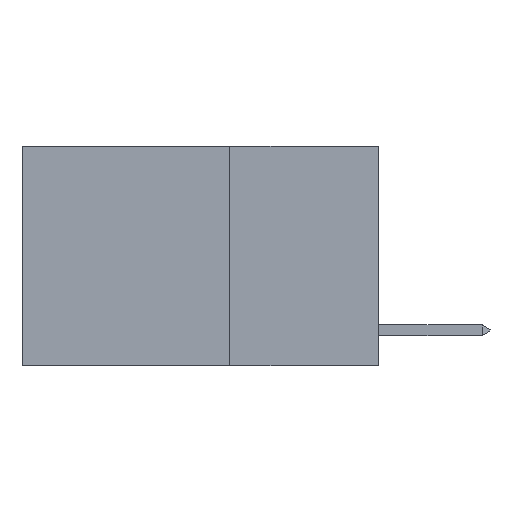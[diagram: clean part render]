
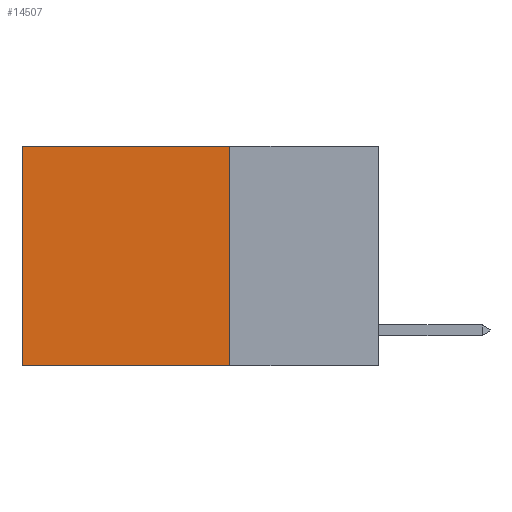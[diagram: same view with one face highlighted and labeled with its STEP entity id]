
A CAD part, left-side view. The second image highlights one B-rep face of the part: STEP entity #14507.
In plain terms, the highlighted planar face has unit normal (-1, 0, 0).
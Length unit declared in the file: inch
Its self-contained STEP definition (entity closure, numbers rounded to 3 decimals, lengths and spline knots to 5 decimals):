
#401 = DIRECTION ( 'NONE',  ( 0., 1., 0. ) ) ;
#1556 = ORIENTED_EDGE ( 'NONE', *, *, #18446, .T. ) ;
#2147 = CARTESIAN_POINT ( 'NONE',  ( 0.2625, 0.25, 0. ) ) ;
#2982 = VERTEX_POINT ( 'NONE', #14710 ) ;
#4727 = CARTESIAN_POINT ( 'NONE',  ( 0.2625, 0.25, -0.37 ) ) ;
#6183 = ORIENTED_EDGE ( 'NONE', *, *, #27543, .T. ) ;
#8913 = CARTESIAN_POINT ( 'NONE',  ( 0.2625, 0.25, 0. ) ) ;
#9107 = VECTOR ( 'NONE', #10740, 39.37008 ) ;
#9133 = LINE ( 'NONE', #17726, #14796 ) ;
#10447 = CARTESIAN_POINT ( 'NONE',  ( 0.2625, 0.6, 0. ) ) ;
#10517 = EDGE_CURVE ( 'NONE', #2982, #15190, #16819, .T. ) ;
#10740 = DIRECTION ( 'NONE',  ( 0., 1., 0. ) ) ;
#11075 = DIRECTION ( 'NONE',  ( 0., 0., -1. ) ) ;
#11199 = VECTOR ( 'NONE', #13147, 39.37008 ) ;
#11782 = ORIENTED_EDGE ( 'NONE', *, *, #15680, .F. ) ;
#12975 = LINE ( 'NONE', #10447, #17911 ) ;
#13147 = DIRECTION ( 'NONE',  ( 0., 0., -1. ) ) ;
#14507 = ADVANCED_FACE ( 'NONE', ( #14511 ), #19463, .F. ) ;
#14511 = FACE_OUTER_BOUND ( 'NONE', #19646, .T. ) ;
#14710 = CARTESIAN_POINT ( 'NONE',  ( 0.2625, 0.25, 0. ) ) ;
#14771 = LINE ( 'NONE', #19138, #9107 ) ;
#14796 = VECTOR ( 'NONE', #401, 39.37008 ) ;
#15190 = VERTEX_POINT ( 'NONE', #4727 ) ;
#15680 = EDGE_CURVE ( 'NONE', #15190, #26964, #14771, .T. ) ;
#16819 = LINE ( 'NONE', #2147, #11199 ) ;
#17726 = CARTESIAN_POINT ( 'NONE',  ( 0.2625, 0.25, 0. ) ) ;
#17911 = VECTOR ( 'NONE', #18948, 39.37008 ) ;
#18446 = EDGE_CURVE ( 'NONE', #2982, #23501, #9133, .T. ) ;
#18948 = DIRECTION ( 'NONE',  ( 0., 0., -1. ) ) ;
#19138 = CARTESIAN_POINT ( 'NONE',  ( 0.2625, 0.25, -0.37 ) ) ;
#19463 = PLANE ( 'NONE',  #19617 ) ;
#19617 = AXIS2_PLACEMENT_3D ( 'NONE', #8913, #23607, #11075 ) ;
#19646 = EDGE_LOOP ( 'NONE', ( #6183, #11782, #19847, #1556 ) ) ;
#19847 = ORIENTED_EDGE ( 'NONE', *, *, #10517, .F. ) ;
#23501 = VERTEX_POINT ( 'NONE', #27361 ) ;
#23607 = DIRECTION ( 'NONE',  ( 1., 0., 0. ) ) ;
#24385 = CARTESIAN_POINT ( 'NONE',  ( 0.2625, 0.6, -0.37 ) ) ;
#26964 = VERTEX_POINT ( 'NONE', #24385 ) ;
#27361 = CARTESIAN_POINT ( 'NONE',  ( 0.2625, 0.6, 0. ) ) ;
#27543 = EDGE_CURVE ( 'NONE', #23501, #26964, #12975, .T. ) ;
